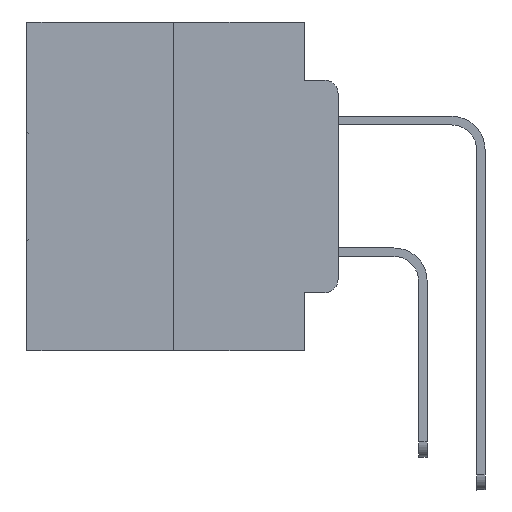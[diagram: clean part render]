
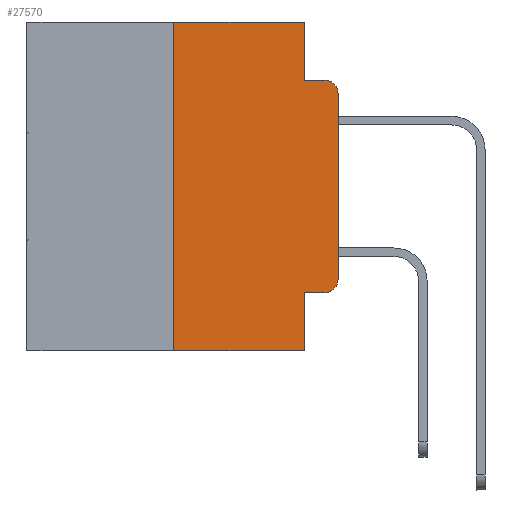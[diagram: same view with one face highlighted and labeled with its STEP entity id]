
A CAD part, left-side view. The second image highlights one B-rep face of the part: STEP entity #27570.
In plain terms, the highlighted planar face has unit normal (-1, 0, 0).
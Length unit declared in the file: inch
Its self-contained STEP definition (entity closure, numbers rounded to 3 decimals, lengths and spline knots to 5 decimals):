
#482 = DIRECTION ( 'NONE',  ( 0., 0., 1. ) ) ;
#557 = DIRECTION ( 'NONE',  ( 0., 0., -1. ) ) ;
#576 = DIRECTION ( 'NONE',  ( 0., 0., -1. ) ) ;
#665 = CARTESIAN_POINT ( 'NONE',  ( 0., 0.051, 0. ) ) ;
#1144 = CARTESIAN_POINT ( 'NONE',  ( 0., 0.473, 0. ) ) ;
#1375 = LINE ( 'NONE', #20160, #23237 ) ;
#1662 = CARTESIAN_POINT ( 'NONE',  ( 0., 0.25, 0. ) ) ;
#1817 = ORIENTED_EDGE ( 'NONE', *, *, #16459, .F. ) ;
#2316 = LINE ( 'NONE', #30947, #9092 ) ;
#3419 = ORIENTED_EDGE ( 'NONE', *, *, #28207, .F. ) ;
#3649 = EDGE_CURVE ( 'NONE', #17343, #17445, #26359, .T. ) ;
#4060 = VERTEX_POINT ( 'NONE', #24112 ) ;
#4102 = CIRCLE ( 'NONE', #25470, 0.02 ) ;
#4493 = EDGE_CURVE ( 'NONE', #31522, #30862, #4102, .T. ) ;
#4606 = DIRECTION ( 'NONE',  ( 0., -1., 0. ) ) ;
#4907 = LINE ( 'NONE', #665, #32458 ) ;
#4948 = DIRECTION ( 'NONE',  ( 0., -1., 0. ) ) ;
#5044 = ORIENTED_EDGE ( 'NONE', *, *, #3649, .T. ) ;
#5365 = CARTESIAN_POINT ( 'NONE',  ( 0., 0.473, 0. ) ) ;
#5385 = EDGE_CURVE ( 'NONE', #17445, #21677, #10924, .T. ) ;
#6283 = DIRECTION ( 'NONE',  ( 0., 0., -1. ) ) ;
#7002 = ORIENTED_EDGE ( 'NONE', *, *, #4493, .T. ) ;
#7632 = VERTEX_POINT ( 'NONE', #25811 ) ;
#7896 = DIRECTION ( 'NONE',  ( 0., -1., 0. ) ) ;
#9092 = VECTOR ( 'NONE', #482, 39.37008 ) ;
#10835 = CARTESIAN_POINT ( 'NONE',  ( 0., 0.02, -0.0885 ) ) ;
#10924 = CIRCLE ( 'NONE', #30264, 0.02 ) ;
#11114 = CARTESIAN_POINT ( 'NONE',  ( 0., 0., -0.1085 ) ) ;
#11312 = VERTEX_POINT ( 'NONE', #23249 ) ;
#12524 = VECTOR ( 'NONE', #21987, 39.37008 ) ;
#12658 = VECTOR ( 'NONE', #7896, 39.37008 ) ;
#13439 = EDGE_CURVE ( 'NONE', #4060, #31078, #26826, .T. ) ;
#14587 = VERTEX_POINT ( 'NONE', #23994 ) ;
#14589 = ORIENTED_EDGE ( 'NONE', *, *, #14733, .F. ) ;
#14684 = DIRECTION ( 'NONE',  ( -1., 0., 0. ) ) ;
#14733 = EDGE_CURVE ( 'NONE', #11312, #30862, #1375, .T. ) ;
#14734 = CARTESIAN_POINT ( 'NONE',  ( 0., 0.051, -0.4115 ) ) ;
#15392 = ORIENTED_EDGE ( 'NONE', *, *, #32643, .F. ) ;
#15705 = CARTESIAN_POINT ( 'NONE',  ( 0., 0.051, -0.4115 ) ) ;
#15843 = DIRECTION ( 'NONE',  ( -1., 0., 0. ) ) ;
#16062 = EDGE_LOOP ( 'NONE', ( #19753, #7002, #14589, #1817, #15392, #3419, #16989, #24443, #5044, #25224 ) ) ;
#16430 = PLANE ( 'NONE',  #23732 ) ;
#16459 = EDGE_CURVE ( 'NONE', #7632, #11312, #24327, .T. ) ;
#16989 = ORIENTED_EDGE ( 'NONE', *, *, #13439, .T. ) ;
#17343 = VERTEX_POINT ( 'NONE', #15705 ) ;
#17445 = VERTEX_POINT ( 'NONE', #28647 ) ;
#19698 = VECTOR ( 'NONE', #4606, 39.37008 ) ;
#19753 = ORIENTED_EDGE ( 'NONE', *, *, #32125, .T. ) ;
#20160 = CARTESIAN_POINT ( 'NONE',  ( 0., 0.051, -0.0885 ) ) ;
#21491 = DIRECTION ( 'NONE',  ( 1., 0., 0. ) ) ;
#21677 = VERTEX_POINT ( 'NONE', #27406 ) ;
#21987 = DIRECTION ( 'NONE',  ( 0., 0., 1. ) ) ;
#23237 = VECTOR ( 'NONE', #4948, 39.37008 ) ;
#23249 = CARTESIAN_POINT ( 'NONE',  ( 0., 0.051, -0.0885 ) ) ;
#23563 = VECTOR ( 'NONE', #31914, 39.37008 ) ;
#23732 = AXIS2_PLACEMENT_3D ( 'NONE', #1144, #21491, #6283 ) ;
#23994 = CARTESIAN_POINT ( 'NONE',  ( 0., 0.25, 0. ) ) ;
#24112 = CARTESIAN_POINT ( 'NONE',  ( 0., 0.25, -0.5 ) ) ;
#24327 = LINE ( 'NONE', #29436, #23563 ) ;
#24443 = ORIENTED_EDGE ( 'NONE', *, *, #29839, .F. ) ;
#24495 = DIRECTION ( 'NONE',  ( 0., -1., 0. ) ) ;
#25224 = ORIENTED_EDGE ( 'NONE', *, *, #5385, .T. ) ;
#25470 = AXIS2_PLACEMENT_3D ( 'NONE', #30820, #15843, #576 ) ;
#25583 = FACE_OUTER_BOUND ( 'NONE', #16062, .T. ) ;
#25811 = CARTESIAN_POINT ( 'NONE',  ( 0., 0.051, 0. ) ) ;
#26359 = LINE ( 'NONE', #14734, #19698 ) ;
#26826 = LINE ( 'NONE', #31980, #29156 ) ;
#27406 = CARTESIAN_POINT ( 'NONE',  ( 0., 0., -0.3915 ) ) ;
#27570 = ADVANCED_FACE ( 'NONE', ( #25583 ), #16430, .F. ) ;
#28207 = EDGE_CURVE ( 'NONE', #4060, #14587, #32508, .T. ) ;
#28647 = CARTESIAN_POINT ( 'NONE',  ( 0., 0.02, -0.4115 ) ) ;
#29156 = VECTOR ( 'NONE', #24495, 39.37008 ) ;
#29436 = CARTESIAN_POINT ( 'NONE',  ( 0., 0.051, 0. ) ) ;
#29691 = CARTESIAN_POINT ( 'NONE',  ( 0., 0.02, -0.3915 ) ) ;
#29839 = EDGE_CURVE ( 'NONE', #17343, #31078, #4907, .T. ) ;
#30264 = AXIS2_PLACEMENT_3D ( 'NONE', #29691, #14684, #32183 ) ;
#30820 = CARTESIAN_POINT ( 'NONE',  ( 0., 0.02, -0.1085 ) ) ;
#30862 = VERTEX_POINT ( 'NONE', #10835 ) ;
#30947 = CARTESIAN_POINT ( 'NONE',  ( 0., 0., 0. ) ) ;
#31078 = VERTEX_POINT ( 'NONE', #31857 ) ;
#31522 = VERTEX_POINT ( 'NONE', #11114 ) ;
#31857 = CARTESIAN_POINT ( 'NONE',  ( 0., 0.051, -0.5 ) ) ;
#31914 = DIRECTION ( 'NONE',  ( 0., 0., -1. ) ) ;
#31980 = CARTESIAN_POINT ( 'NONE',  ( 0., 0.473, -0.5 ) ) ;
#32125 = EDGE_CURVE ( 'NONE', #21677, #31522, #2316, .T. ) ;
#32183 = DIRECTION ( 'NONE',  ( 0., 0., -1. ) ) ;
#32458 = VECTOR ( 'NONE', #557, 39.37008 ) ;
#32508 = LINE ( 'NONE', #1662, #12524 ) ;
#32641 = LINE ( 'NONE', #5365, #12658 ) ;
#32643 = EDGE_CURVE ( 'NONE', #14587, #7632, #32641, .T. ) ;
